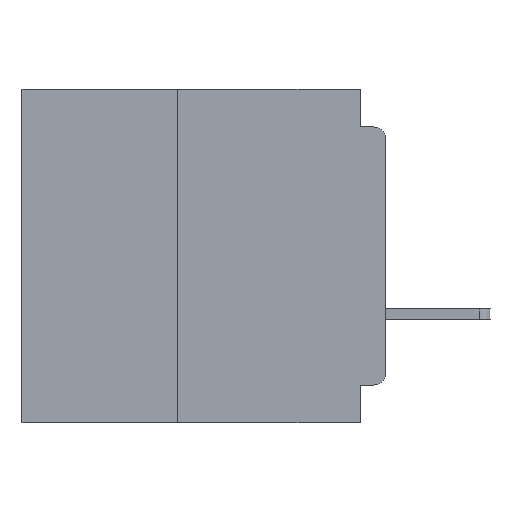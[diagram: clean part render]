
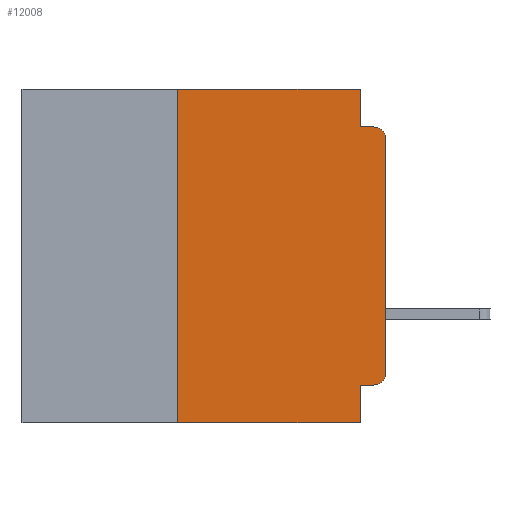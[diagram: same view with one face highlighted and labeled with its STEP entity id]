
A CAD part, left-side view. The second image highlights one B-rep face of the part: STEP entity #12008.
In plain terms, the highlighted planar face has unit normal (-1, 0, 0).
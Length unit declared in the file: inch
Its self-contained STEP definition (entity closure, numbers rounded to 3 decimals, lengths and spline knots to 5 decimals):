
#313 = CARTESIAN_POINT ( 'NONE',  ( 0., 0., -0.34 ) ) ;
#1248 = LINE ( 'NONE', #33001, #26626 ) ;
#1492 = DIRECTION ( 'NONE',  ( 0., -1., 0. ) ) ;
#2224 = DIRECTION ( 'NONE',  ( 1., 0., 0. ) ) ;
#2589 = VECTOR ( 'NONE', #12719, 39.37008 ) ;
#2635 = DIRECTION ( 'NONE',  ( 0., 0., 1. ) ) ;
#3939 = LINE ( 'NONE', #19906, #29298 ) ;
#5401 = CARTESIAN_POINT ( 'NONE',  ( 0., 0.015, -0.06 ) ) ;
#6131 = ORIENTED_EDGE ( 'NONE', *, *, #20724, .T. ) ;
#7003 = CARTESIAN_POINT ( 'NONE',  ( 0., 0.031, 0. ) ) ;
#7229 = VERTEX_POINT ( 'NONE', #53907 ) ;
#7285 = ORIENTED_EDGE ( 'NONE', *, *, #65333, .T. ) ;
#7601 = CARTESIAN_POINT ( 'NONE',  ( 0., 0., -0.045 ) ) ;
#8326 = LINE ( 'NONE', #38875, #45493 ) ;
#9687 = ORIENTED_EDGE ( 'NONE', *, *, #40705, .F. ) ;
#9987 = AXIS2_PLACEMENT_3D ( 'NONE', #12210, #2224, #37611 ) ;
#10533 = DIRECTION ( 'NONE',  ( 0., 0., -1. ) ) ;
#11478 = CARTESIAN_POINT ( 'NONE',  ( 0., 0.031, -0.045 ) ) ;
#12008 = ADVANCED_FACE ( 'NONE', ( #12662 ), #32589, .F. ) ;
#12210 = CARTESIAN_POINT ( 'NONE',  ( 0., 0.437, 0. ) ) ;
#12504 = CIRCLE ( 'NONE', #63384, 0.015 ) ;
#12662 = FACE_OUTER_BOUND ( 'NONE', #38460, .T. ) ;
#12719 = DIRECTION ( 'NONE',  ( 0., -1., 0. ) ) ;
#13371 = VERTEX_POINT ( 'NONE', #63501 ) ;
#15529 = CARTESIAN_POINT ( 'NONE',  ( 0., 0.437, 0. ) ) ;
#15562 = EDGE_CURVE ( 'NONE', #32237, #33846, #8326, .T. ) ;
#17669 = CIRCLE ( 'NONE', #49835, 0.015 ) ;
#17789 = CARTESIAN_POINT ( 'NONE',  ( 0., 0.015, -0.045 ) ) ;
#18431 = ORIENTED_EDGE ( 'NONE', *, *, #63377, .F. ) ;
#18984 = DIRECTION ( 'NONE',  ( 0., 0., -1. ) ) ;
#19906 = CARTESIAN_POINT ( 'NONE',  ( 0., 0., -0.355 ) ) ;
#20724 = EDGE_CURVE ( 'NONE', #41620, #42002, #44051, .T. ) ;
#21433 = ORIENTED_EDGE ( 'NONE', *, *, #52783, .F. ) ;
#21656 = CARTESIAN_POINT ( 'NONE',  ( 0., 0.437, -0.4 ) ) ;
#23834 = EDGE_CURVE ( 'NONE', #42002, #27248, #12504, .T. ) ;
#24178 = CARTESIAN_POINT ( 'NONE',  ( 0., 0.031, -0.4 ) ) ;
#24957 = VECTOR ( 'NONE', #31972, 39.37008 ) ;
#26463 = ORIENTED_EDGE ( 'NONE', *, *, #23834, .T. ) ;
#26626 = VECTOR ( 'NONE', #2635, 39.37008 ) ;
#27244 = EDGE_CURVE ( 'NONE', #33846, #27248, #31161, .T. ) ;
#27248 = VERTEX_POINT ( 'NONE', #17789 ) ;
#28112 = LINE ( 'NONE', #32181, #24957 ) ;
#28168 = DIRECTION ( 'NONE',  ( -1., 0., 0. ) ) ;
#28849 = CARTESIAN_POINT ( 'NONE',  ( 0., 0.031, -0.355 ) ) ;
#29077 = VECTOR ( 'NONE', #56408, 39.37008 ) ;
#29298 = VECTOR ( 'NONE', #50112, 39.37008 ) ;
#31161 = LINE ( 'NONE', #7601, #2589 ) ;
#31972 = DIRECTION ( 'NONE',  ( 0., 0., -1. ) ) ;
#32181 = CARTESIAN_POINT ( 'NONE',  ( 0., 0.031, -0.4 ) ) ;
#32237 = VERTEX_POINT ( 'NONE', #7003 ) ;
#32589 = PLANE ( 'NONE',  #9987 ) ;
#33001 = CARTESIAN_POINT ( 'NONE',  ( 0., 0.25, -0.4 ) ) ;
#33846 = VERTEX_POINT ( 'NONE', #11478 ) ;
#34978 = EDGE_CURVE ( 'NONE', #63247, #32237, #44342, .T. ) ;
#36130 = CARTESIAN_POINT ( 'NONE',  ( 0., 0., 0. ) ) ;
#37611 = DIRECTION ( 'NONE',  ( 0., 0., -1. ) ) ;
#38460 = EDGE_LOOP ( 'NONE', ( #6131, #26463, #44511, #58977, #55376, #9687, #7285, #18431, #21433, #48556 ) ) ;
#38875 = CARTESIAN_POINT ( 'NONE',  ( 0., 0.031, 0. ) ) ;
#40705 = EDGE_CURVE ( 'NONE', #13371, #63247, #1248, .T. ) ;
#40773 = DIRECTION ( 'NONE',  ( -1., 0., 0. ) ) ;
#41620 = VERTEX_POINT ( 'NONE', #313 ) ;
#42002 = VERTEX_POINT ( 'NONE', #58661 ) ;
#42733 = VECTOR ( 'NONE', #45802, 39.37008 ) ;
#43923 = VERTEX_POINT ( 'NONE', #28849 ) ;
#44051 = LINE ( 'NONE', #36130, #29077 ) ;
#44342 = LINE ( 'NONE', #15529, #42733 ) ;
#44511 = ORIENTED_EDGE ( 'NONE', *, *, #27244, .F. ) ;
#45493 = VECTOR ( 'NONE', #18984, 39.37008 ) ;
#45751 = EDGE_CURVE ( 'NONE', #7229, #41620, #17669, .T. ) ;
#45802 = DIRECTION ( 'NONE',  ( 0., -1., 0. ) ) ;
#45864 = VERTEX_POINT ( 'NONE', #24178 ) ;
#48556 = ORIENTED_EDGE ( 'NONE', *, *, #45751, .T. ) ;
#49835 = AXIS2_PLACEMENT_3D ( 'NONE', #58403, #28168, #63467 ) ;
#50112 = DIRECTION ( 'NONE',  ( 0., 1., 0. ) ) ;
#50670 = VECTOR ( 'NONE', #1492, 39.37008 ) ;
#52250 = LINE ( 'NONE', #21656, #50670 ) ;
#52783 = EDGE_CURVE ( 'NONE', #7229, #43923, #3939, .T. ) ;
#53907 = CARTESIAN_POINT ( 'NONE',  ( 0., 0.015, -0.355 ) ) ;
#55376 = ORIENTED_EDGE ( 'NONE', *, *, #34978, .F. ) ;
#56219 = CARTESIAN_POINT ( 'NONE',  ( 0., 0.25, 0. ) ) ;
#56408 = DIRECTION ( 'NONE',  ( 0., 0., 1. ) ) ;
#58403 = CARTESIAN_POINT ( 'NONE',  ( 0., 0.015, -0.34 ) ) ;
#58661 = CARTESIAN_POINT ( 'NONE',  ( 0., 0., -0.06 ) ) ;
#58977 = ORIENTED_EDGE ( 'NONE', *, *, #15562, .F. ) ;
#63247 = VERTEX_POINT ( 'NONE', #56219 ) ;
#63377 = EDGE_CURVE ( 'NONE', #43923, #45864, #28112, .T. ) ;
#63384 = AXIS2_PLACEMENT_3D ( 'NONE', #5401, #40773, #10533 ) ;
#63467 = DIRECTION ( 'NONE',  ( 0., 0., -1. ) ) ;
#63501 = CARTESIAN_POINT ( 'NONE',  ( 0., 0.25, -0.4 ) ) ;
#65333 = EDGE_CURVE ( 'NONE', #13371, #45864, #52250, .T. ) ;
